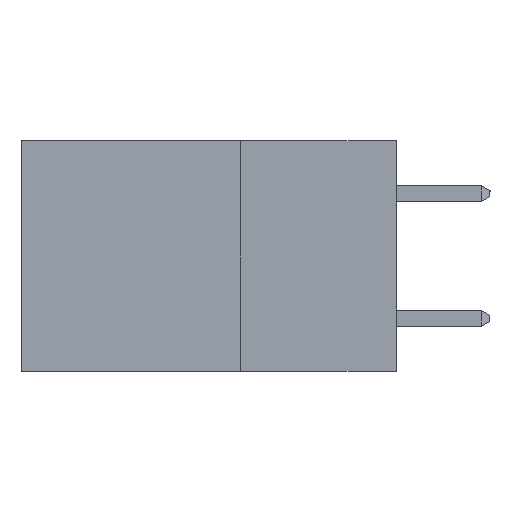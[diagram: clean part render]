
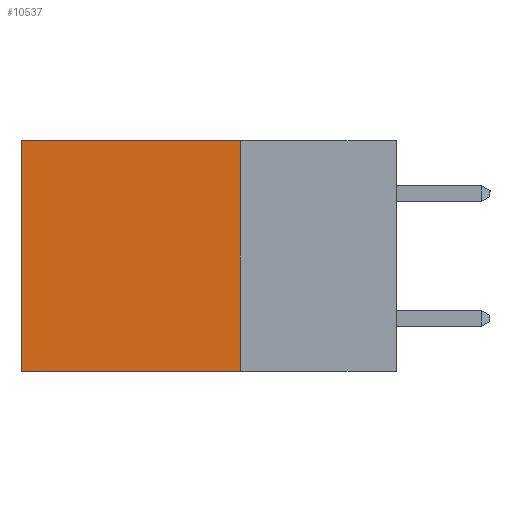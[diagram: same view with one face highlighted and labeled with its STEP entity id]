
A CAD part, left-side view. The second image highlights one B-rep face of the part: STEP entity #10537.
In plain terms, the highlighted planar face has unit normal (-1, 0, 0).
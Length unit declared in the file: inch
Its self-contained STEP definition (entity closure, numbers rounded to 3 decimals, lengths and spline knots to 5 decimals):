
#409 = VERTEX_POINT ( 'NONE', #16898 ) ;
#2396 = DIRECTION ( 'NONE',  ( 1., 0., 0. ) ) ;
#2704 = CARTESIAN_POINT ( 'NONE',  ( 0.2615, 0.25, 0. ) ) ;
#3667 = VERTEX_POINT ( 'NONE', #3749 ) ;
#3684 = LINE ( 'NONE', #13251, #16674 ) ;
#3749 = CARTESIAN_POINT ( 'NONE',  ( 0.2615, 0.25, 0. ) ) ;
#4013 = VERTEX_POINT ( 'NONE', #17578 ) ;
#5414 = DIRECTION ( 'NONE',  ( 0., 0., -1. ) ) ;
#5826 = PLANE ( 'NONE',  #14842 ) ;
#6141 = VECTOR ( 'NONE', #20201, 39.37008 ) ;
#6757 = EDGE_CURVE ( 'NONE', #3667, #4013, #8644, .T. ) ;
#8644 = LINE ( 'NONE', #2704, #6141 ) ;
#8752 = ORIENTED_EDGE ( 'NONE', *, *, #17855, .F. ) ;
#9295 = ORIENTED_EDGE ( 'NONE', *, *, #6757, .T. ) ;
#10101 = LINE ( 'NONE', #15317, #12614 ) ;
#10130 = EDGE_CURVE ( 'NONE', #14601, #409, #16987, .T. ) ;
#10133 = DIRECTION ( 'NONE',  ( 0., 0., -1. ) ) ;
#10400 = CARTESIAN_POINT ( 'NONE',  ( 0.2615, 0.25, -0.37 ) ) ;
#10501 = FACE_OUTER_BOUND ( 'NONE', #14491, .T. ) ;
#10537 = ADVANCED_FACE ( 'NONE', ( #10501 ), #5826, .F. ) ;
#12393 = ORIENTED_EDGE ( 'NONE', *, *, #16484, .T. ) ;
#12614 = VECTOR ( 'NONE', #13328, 39.37008 ) ;
#12838 = VECTOR ( 'NONE', #15012, 39.37008 ) ;
#13251 = CARTESIAN_POINT ( 'NONE',  ( 0.2615, 0.25, -0.37 ) ) ;
#13328 = DIRECTION ( 'NONE',  ( 0., 0., -1. ) ) ;
#13833 = CARTESIAN_POINT ( 'NONE',  ( 0.2615, 0.25, -0.37 ) ) ;
#14491 = EDGE_LOOP ( 'NONE', ( #12393, #16935, #8752, #9295 ) ) ;
#14601 = VERTEX_POINT ( 'NONE', #16708 ) ;
#14842 = AXIS2_PLACEMENT_3D ( 'NONE', #10400, #2396, #5414 ) ;
#15012 = DIRECTION ( 'NONE',  ( 0., 1., 0. ) ) ;
#15317 = CARTESIAN_POINT ( 'NONE',  ( 0.2615, 0.6, -0.37 ) ) ;
#16484 = EDGE_CURVE ( 'NONE', #4013, #409, #10101, .T. ) ;
#16674 = VECTOR ( 'NONE', #10133, 39.37008 ) ;
#16708 = CARTESIAN_POINT ( 'NONE',  ( 0.2615, 0.25, -0.37 ) ) ;
#16898 = CARTESIAN_POINT ( 'NONE',  ( 0.2615, 0.6, -0.37 ) ) ;
#16935 = ORIENTED_EDGE ( 'NONE', *, *, #10130, .F. ) ;
#16987 = LINE ( 'NONE', #13833, #12838 ) ;
#17578 = CARTESIAN_POINT ( 'NONE',  ( 0.2615, 0.6, 0. ) ) ;
#17855 = EDGE_CURVE ( 'NONE', #3667, #14601, #3684, .T. ) ;
#20201 = DIRECTION ( 'NONE',  ( 0., 1., 0. ) ) ;
